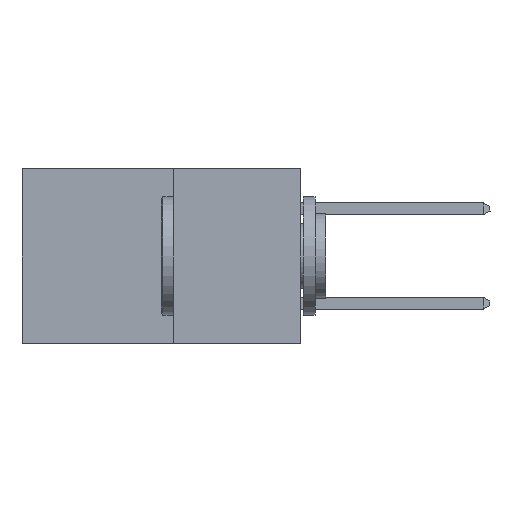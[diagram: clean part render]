
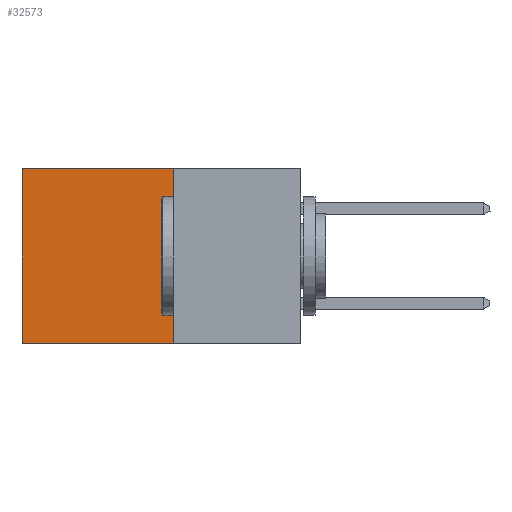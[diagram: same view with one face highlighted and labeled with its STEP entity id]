
A CAD part, left-side view. The second image highlights one B-rep face of the part: STEP entity #32573.
In plain terms, the highlighted planar face has unit normal (-1, 0, 0).
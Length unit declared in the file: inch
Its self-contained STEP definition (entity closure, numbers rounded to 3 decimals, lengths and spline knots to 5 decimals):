
#2443 = LINE ( 'NONE', #13479, #16271 ) ;
#2516 = VERTEX_POINT ( 'NONE', #20913 ) ;
#3703 = LINE ( 'NONE', #29787, #23626 ) ;
#7392 = AXIS2_PLACEMENT_3D ( 'NONE', #17133, #24926, #9361 ) ;
#8505 = EDGE_CURVE ( 'NONE', #2516, #16451, #2443, .T. ) ;
#8550 = EDGE_CURVE ( 'NONE', #2516, #10297, #22380, .T. ) ;
#8688 = EDGE_CURVE ( 'NONE', #10297, #24707, #30287, .T. ) ;
#9361 = DIRECTION ( 'NONE',  ( 0., 0., -1. ) ) ;
#10297 = VERTEX_POINT ( 'NONE', #11901 ) ;
#10614 = ORIENTED_EDGE ( 'NONE', *, *, #20698, .F. ) ;
#11434 = CARTESIAN_POINT ( 'NONE',  ( 0.277, 0.59, -0.37 ) ) ;
#11879 = PLANE ( 'NONE',  #7392 ) ;
#11901 = CARTESIAN_POINT ( 'NONE',  ( 0.277, 0.59, 0. ) ) ;
#13479 = CARTESIAN_POINT ( 'NONE',  ( 0.277, 0.27, -0.37 ) ) ;
#14640 = VECTOR ( 'NONE', #26448, 39.37008 ) ;
#15135 = CARTESIAN_POINT ( 'NONE',  ( 0.277, 0.27, -0.37 ) ) ;
#16271 = VECTOR ( 'NONE', #28895, 39.37008 ) ;
#16451 = VERTEX_POINT ( 'NONE', #15135 ) ;
#16677 = DIRECTION ( 'NONE',  ( 0., 0., -1. ) ) ;
#17133 = CARTESIAN_POINT ( 'NONE',  ( 0.277, 0.27, -0.37 ) ) ;
#18307 = EDGE_LOOP ( 'NONE', ( #26218, #10614, #28291, #27236 ) ) ;
#18749 = CARTESIAN_POINT ( 'NONE',  ( 0.277, 0.27, 0. ) ) ;
#20465 = FACE_OUTER_BOUND ( 'NONE', #18307, .T. ) ;
#20698 = EDGE_CURVE ( 'NONE', #16451, #24707, #3703, .T. ) ;
#20788 = CARTESIAN_POINT ( 'NONE',  ( 0.277, 0.59, -0.37 ) ) ;
#20913 = CARTESIAN_POINT ( 'NONE',  ( 0.277, 0.27, 0. ) ) ;
#22380 = LINE ( 'NONE', #18749, #14640 ) ;
#23559 = VECTOR ( 'NONE', #16677, 39.37008 ) ;
#23626 = VECTOR ( 'NONE', #32284, 39.37008 ) ;
#24707 = VERTEX_POINT ( 'NONE', #20788 ) ;
#24926 = DIRECTION ( 'NONE',  ( 1., 0., 0. ) ) ;
#26218 = ORIENTED_EDGE ( 'NONE', *, *, #8688, .T. ) ;
#26448 = DIRECTION ( 'NONE',  ( 0., 1., 0. ) ) ;
#27236 = ORIENTED_EDGE ( 'NONE', *, *, #8550, .T. ) ;
#28291 = ORIENTED_EDGE ( 'NONE', *, *, #8505, .F. ) ;
#28895 = DIRECTION ( 'NONE',  ( 0., 0., -1. ) ) ;
#29787 = CARTESIAN_POINT ( 'NONE',  ( 0.277, 0.27, -0.37 ) ) ;
#30287 = LINE ( 'NONE', #11434, #23559 ) ;
#32284 = DIRECTION ( 'NONE',  ( 0., 1., 0. ) ) ;
#32573 = ADVANCED_FACE ( 'NONE', ( #20465 ), #11879, .F. ) ;
